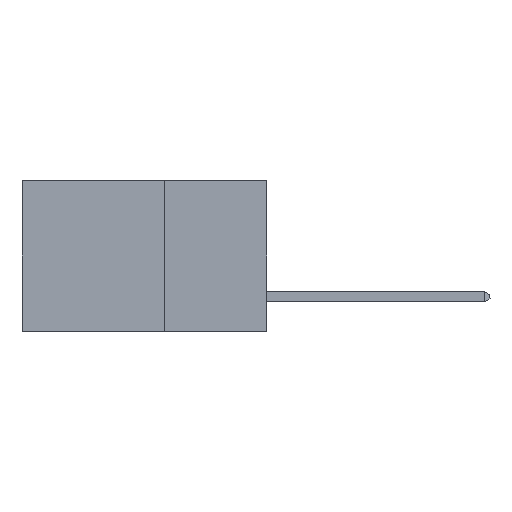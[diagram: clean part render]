
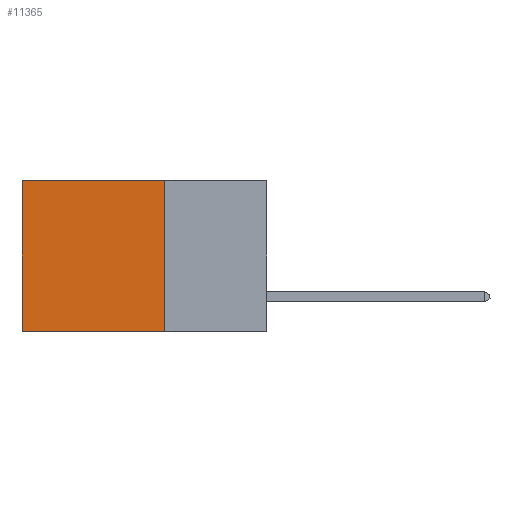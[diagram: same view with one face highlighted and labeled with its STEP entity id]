
A CAD part, left-side view. The second image highlights one B-rep face of the part: STEP entity #11365.
In plain terms, the highlighted planar face has unit normal (-1, 0, 0).
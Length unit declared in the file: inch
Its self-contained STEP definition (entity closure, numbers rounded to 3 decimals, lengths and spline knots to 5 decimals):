
#118 = DIRECTION ( 'NONE',  ( 1., 0., 0. ) ) ;
#470 = DIRECTION ( 'NONE',  ( 0., 1., 0. ) ) ;
#614 = AXIS2_PLACEMENT_3D ( 'NONE', #27116, #118, #15885 ) ;
#2129 = LINE ( 'NONE', #4848, #6773 ) ;
#2336 = VECTOR ( 'NONE', #8151, 39.37008 ) ;
#2949 = VERTEX_POINT ( 'NONE', #12262 ) ;
#3073 = LINE ( 'NONE', #19276, #2336 ) ;
#3378 = CARTESIAN_POINT ( 'NONE',  ( 0.2875, 0.25, 0. ) ) ;
#4848 = CARTESIAN_POINT ( 'NONE',  ( 0.2875, 0.25, 0. ) ) ;
#5268 = LINE ( 'NONE', #28626, #23890 ) ;
#6773 = VECTOR ( 'NONE', #18351, 39.37008 ) ;
#7609 = CARTESIAN_POINT ( 'NONE',  ( 0.2875, 0.25, -0.37 ) ) ;
#7983 = VERTEX_POINT ( 'NONE', #20885 ) ;
#8005 = VERTEX_POINT ( 'NONE', #7609 ) ;
#8038 = ORIENTED_EDGE ( 'NONE', *, *, #16360, .T. ) ;
#8151 = DIRECTION ( 'NONE',  ( 0., 0., -1. ) ) ;
#10196 = ORIENTED_EDGE ( 'NONE', *, *, #21519, .F. ) ;
#11365 = ADVANCED_FACE ( 'NONE', ( #22306 ), #11416, .F. ) ;
#11416 = PLANE ( 'NONE',  #614 ) ;
#11739 = VECTOR ( 'NONE', #470, 39.37008 ) ;
#12262 = CARTESIAN_POINT ( 'NONE',  ( 0.2875, 0.6, -0.37 ) ) ;
#15171 = DIRECTION ( 'NONE',  ( 0., 0., -1. ) ) ;
#15201 = EDGE_LOOP ( 'NONE', ( #8038, #28512, #10196, #15935 ) ) ;
#15885 = DIRECTION ( 'NONE',  ( 0., 0., -1. ) ) ;
#15935 = ORIENTED_EDGE ( 'NONE', *, *, #25513, .T. ) ;
#16360 = EDGE_CURVE ( 'NONE', #7983, #2949, #3073, .T. ) ;
#17651 = LINE ( 'NONE', #27442, #11739 ) ;
#18351 = DIRECTION ( 'NONE',  ( 0., 1., 0. ) ) ;
#19276 = CARTESIAN_POINT ( 'NONE',  ( 0.2875, 0.6, 0. ) ) ;
#20885 = CARTESIAN_POINT ( 'NONE',  ( 0.2875, 0.6, 0. ) ) ;
#21519 = EDGE_CURVE ( 'NONE', #23105, #8005, #5268, .T. ) ;
#22306 = FACE_OUTER_BOUND ( 'NONE', #15201, .T. ) ;
#23105 = VERTEX_POINT ( 'NONE', #3378 ) ;
#23890 = VECTOR ( 'NONE', #15171, 39.37008 ) ;
#25513 = EDGE_CURVE ( 'NONE', #23105, #7983, #2129, .T. ) ;
#27116 = CARTESIAN_POINT ( 'NONE',  ( 0.2875, 0.25, 0. ) ) ;
#27392 = EDGE_CURVE ( 'NONE', #8005, #2949, #17651, .T. ) ;
#27442 = CARTESIAN_POINT ( 'NONE',  ( 0.2875, 0.25, -0.37 ) ) ;
#28512 = ORIENTED_EDGE ( 'NONE', *, *, #27392, .F. ) ;
#28626 = CARTESIAN_POINT ( 'NONE',  ( 0.2875, 0.25, 0. ) ) ;
